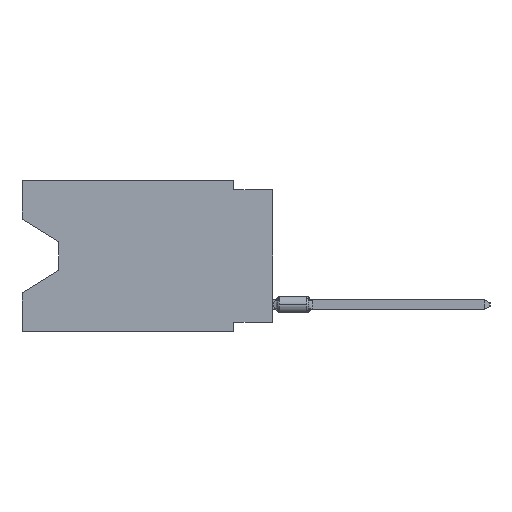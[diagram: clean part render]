
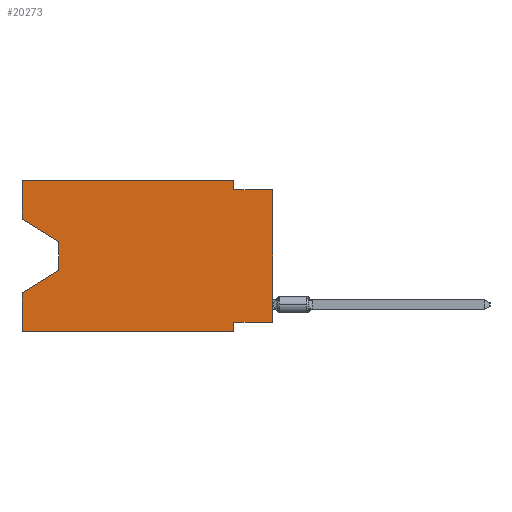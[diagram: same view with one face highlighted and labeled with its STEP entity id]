
A CAD part, left-side view. The second image highlights one B-rep face of the part: STEP entity #20273.
In plain terms, the highlighted planar face has unit normal (-1, 0, 0).
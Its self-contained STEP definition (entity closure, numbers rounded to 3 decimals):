
#759 = VECTOR ( 'NONE', #20123, 1000. ) ;
#1590 = EDGE_CURVE ( 'NONE', #35907, #59548, #45788, .T. ) ;
#1800 = CARTESIAN_POINT ( 'NONE',  ( 0., 13.97, -4.013 ) ) ;
#2818 = VECTOR ( 'NONE', #36669, 1000. ) ;
#3202 = ORIENTED_EDGE ( 'NONE', *, *, #9615, .T. ) ;
#4011 = VERTEX_POINT ( 'NONE', #62140 ) ;
#5389 = VERTEX_POINT ( 'NONE', #10256 ) ;
#5403 = ORIENTED_EDGE ( 'NONE', *, *, #61108, .F. ) ;
#5468 = LINE ( 'NONE', #34675, #48873 ) ;
#5661 = CARTESIAN_POINT ( 'NONE',  ( 0., 13.97, -5.893 ) ) ;
#5824 = VECTOR ( 'NONE', #37308, 1000. ) ;
#6297 = VECTOR ( 'NONE', #56401, 1000. ) ;
#6630 = LINE ( 'NONE', #29356, #18550 ) ;
#7609 = VERTEX_POINT ( 'NONE', #8195 ) ;
#7896 = AXIS2_PLACEMENT_3D ( 'NONE', #59708, #45573, #60029 ) ;
#8195 = CARTESIAN_POINT ( 'NONE',  ( 0., 0., -0.635 ) ) ;
#9555 = LINE ( 'NONE', #19000, #15318 ) ;
#9615 = EDGE_CURVE ( 'NONE', #15232, #59548, #13059, .T. ) ;
#10256 = CARTESIAN_POINT ( 'NONE',  ( 0., 2.54, 0. ) ) ;
#11349 = CARTESIAN_POINT ( 'NONE',  ( 0., 16.383, -2.546 ) ) ;
#11385 = ORIENTED_EDGE ( 'NONE', *, *, #12353, .T. ) ;
#12353 = EDGE_CURVE ( 'NONE', #12927, #7609, #6630, .T. ) ;
#12921 = CARTESIAN_POINT ( 'NONE',  ( 0., 13.97, -4.013 ) ) ;
#12927 = VERTEX_POINT ( 'NONE', #32301 ) ;
#13059 = LINE ( 'NONE', #55464, #6297 ) ;
#14099 = EDGE_CURVE ( 'NONE', #56197, #41619, #35229, .T. ) ;
#14552 = CARTESIAN_POINT ( 'NONE',  ( 0., 16.383, 0. ) ) ;
#14595 = EDGE_CURVE ( 'NONE', #25696, #5389, #43078, .T. ) ;
#14930 = ORIENTED_EDGE ( 'NONE', *, *, #1590, .F. ) ;
#15203 = DIRECTION ( 'NONE',  ( 0., 0., -1. ) ) ;
#15232 = VERTEX_POINT ( 'NONE', #61722 ) ;
#15318 = VECTOR ( 'NONE', #18080, 1000. ) ;
#15434 = DIRECTION ( 'NONE',  ( 0., -1., 0. ) ) ;
#16228 = ORIENTED_EDGE ( 'NONE', *, *, #19988, .T. ) ;
#16267 = CARTESIAN_POINT ( 'NONE',  ( 0., 16.383, -2.546 ) ) ;
#17170 = VERTEX_POINT ( 'NONE', #31724 ) ;
#17503 = CARTESIAN_POINT ( 'NONE',  ( 0., 0., -9.271 ) ) ;
#17859 = EDGE_CURVE ( 'NONE', #4011, #28195, #58727, .T. ) ;
#18080 = DIRECTION ( 'NONE',  ( 0., 0., 1. ) ) ;
#18163 = EDGE_CURVE ( 'NONE', #15232, #28195, #42233, .T. ) ;
#18550 = VECTOR ( 'NONE', #54670, 1000. ) ;
#18788 = ORIENTED_EDGE ( 'NONE', *, *, #18163, .F. ) ;
#19000 = CARTESIAN_POINT ( 'NONE',  ( 0., 16.383, 0. ) ) ;
#19965 = ORIENTED_EDGE ( 'NONE', *, *, #53524, .F. ) ;
#19988 = EDGE_CURVE ( 'NONE', #41619, #4011, #27188, .T. ) ;
#20123 = DIRECTION ( 'NONE',  ( 0., -1., 0. ) ) ;
#20273 = ADVANCED_FACE ( 'NONE', ( #40545 ), #41797, .F. ) ;
#21226 = CARTESIAN_POINT ( 'NONE',  ( 0., 16.383, -7.36 ) ) ;
#24306 = ORIENTED_EDGE ( 'NONE', *, *, #45527, .F. ) ;
#25429 = ORIENTED_EDGE ( 'NONE', *, *, #14595, .F. ) ;
#25696 = VERTEX_POINT ( 'NONE', #47667 ) ;
#26086 = CARTESIAN_POINT ( 'NONE',  ( 0., 0., -0.635 ) ) ;
#26103 = CARTESIAN_POINT ( 'NONE',  ( 0., 2.54, -9.271 ) ) ;
#26561 = CARTESIAN_POINT ( 'NONE',  ( 0., 2.54, -9.906 ) ) ;
#27188 = LINE ( 'NONE', #1800, #55054 ) ;
#27855 = EDGE_LOOP ( 'NONE', ( #57274, #16228, #41098, #18788, #3202, #14930, #52548, #11385, #19965, #5403, #25429, #24306 ) ) ;
#27892 = CARTESIAN_POINT ( 'NONE',  ( 0., 2.54, -9.906 ) ) ;
#28195 = VERTEX_POINT ( 'NONE', #21226 ) ;
#29356 = CARTESIAN_POINT ( 'NONE',  ( 0., 0., 0. ) ) ;
#30522 = DIRECTION ( 'NONE',  ( 0., -0.855, -0.519 ) ) ;
#31060 = VECTOR ( 'NONE', #57583, 1000. ) ;
#31724 = CARTESIAN_POINT ( 'NONE',  ( 0., 2.54, -0.635 ) ) ;
#32301 = CARTESIAN_POINT ( 'NONE',  ( 0., 0., -9.271 ) ) ;
#34675 = CARTESIAN_POINT ( 'NONE',  ( 0., 2.54, 0. ) ) ;
#35057 = VECTOR ( 'NONE', #48690, 1000. ) ;
#35229 = LINE ( 'NONE', #11349, #57832 ) ;
#35907 = VERTEX_POINT ( 'NONE', #26103 ) ;
#36669 = DIRECTION ( 'NONE',  ( 0., 1., 0. ) ) ;
#37308 = DIRECTION ( 'NONE',  ( 0., 0., -1. ) ) ;
#40545 = FACE_OUTER_BOUND ( 'NONE', #27855, .T. ) ;
#41098 = ORIENTED_EDGE ( 'NONE', *, *, #17859, .T. ) ;
#41619 = VERTEX_POINT ( 'NONE', #12921 ) ;
#41797 = PLANE ( 'NONE',  #7896 ) ;
#42233 = LINE ( 'NONE', #14552, #31060 ) ;
#43078 = LINE ( 'NONE', #58461, #49988 ) ;
#45527 = EDGE_CURVE ( 'NONE', #56197, #25696, #9555, .T. ) ;
#45573 = DIRECTION ( 'NONE',  ( 1., 0., 0. ) ) ;
#45788 = LINE ( 'NONE', #27892, #5824 ) ;
#47667 = CARTESIAN_POINT ( 'NONE',  ( 0., 16.383, 0. ) ) ;
#48690 = DIRECTION ( 'NONE',  ( 0., 0.855, -0.519 ) ) ;
#48873 = VECTOR ( 'NONE', #15203, 1000. ) ;
#49988 = VECTOR ( 'NONE', #15434, 1000. ) ;
#52548 = ORIENTED_EDGE ( 'NONE', *, *, #54174, .F. ) ;
#53524 = EDGE_CURVE ( 'NONE', #17170, #7609, #54325, .T. ) ;
#54174 = EDGE_CURVE ( 'NONE', #12927, #35907, #60538, .T. ) ;
#54325 = LINE ( 'NONE', #26086, #759 ) ;
#54670 = DIRECTION ( 'NONE',  ( 0., 0., 1. ) ) ;
#55054 = VECTOR ( 'NONE', #55743, 1000. ) ;
#55464 = CARTESIAN_POINT ( 'NONE',  ( 0., 16.383, -9.906 ) ) ;
#55743 = DIRECTION ( 'NONE',  ( 0., 0., -1. ) ) ;
#56197 = VERTEX_POINT ( 'NONE', #16267 ) ;
#56401 = DIRECTION ( 'NONE',  ( 0., -1., 0. ) ) ;
#57274 = ORIENTED_EDGE ( 'NONE', *, *, #14099, .T. ) ;
#57583 = DIRECTION ( 'NONE',  ( 0., 0., 1. ) ) ;
#57832 = VECTOR ( 'NONE', #30522, 1000. ) ;
#58461 = CARTESIAN_POINT ( 'NONE',  ( 0., 16.383, 0. ) ) ;
#58727 = LINE ( 'NONE', #5661, #35057 ) ;
#59548 = VERTEX_POINT ( 'NONE', #26561 ) ;
#59708 = CARTESIAN_POINT ( 'NONE',  ( 0., 16.383, 0. ) ) ;
#60029 = DIRECTION ( 'NONE',  ( 0., 0., -1. ) ) ;
#60538 = LINE ( 'NONE', #17503, #2818 ) ;
#61108 = EDGE_CURVE ( 'NONE', #5389, #17170, #5468, .T. ) ;
#61722 = CARTESIAN_POINT ( 'NONE',  ( 0., 16.383, -9.906 ) ) ;
#62140 = CARTESIAN_POINT ( 'NONE',  ( 0., 13.97, -5.893 ) ) ;
